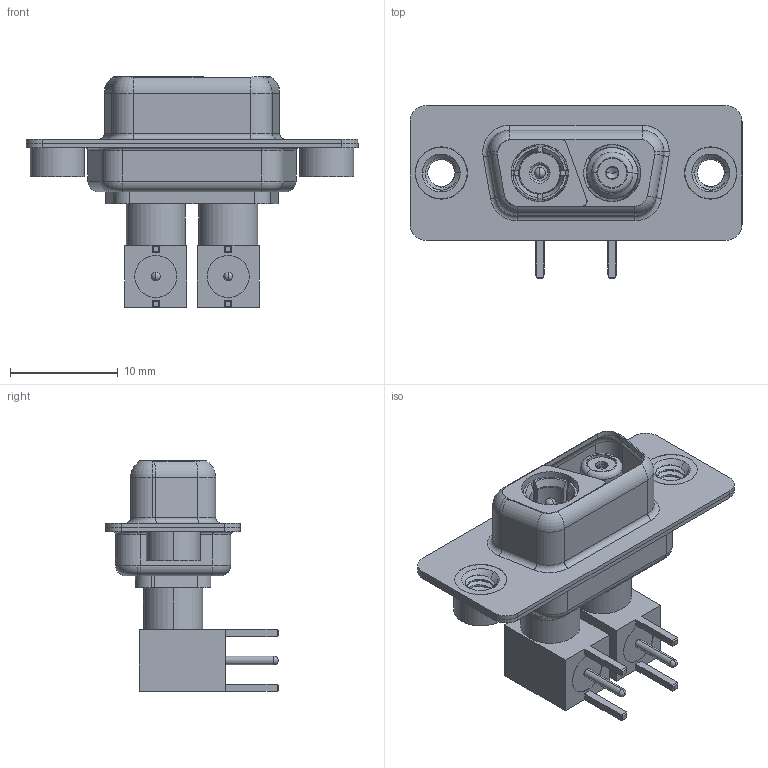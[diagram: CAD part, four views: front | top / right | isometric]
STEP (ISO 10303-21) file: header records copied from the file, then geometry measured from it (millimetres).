
FILE_DESCRIPTION (( 'STEP AP203' ), '1' );
FILE_NAME ('630-2WK2240-7TA.STEP', '2022-05-26T23:52:27', ( '' ), ( '' ), 'SwSTEP 2.0', 'SolidWorks 2020', '' );
FILE_SCHEMA (( 'CONFIG_CONTROL_DESIGN' ));
Length unit declared in the file: millimetre
Products named in the file (17): Locking Collar; 630Combo Shell Front_09 Contacts; 630Combo Housing_2WK2; Co-Ax Jack Assy_RA; Co-Ax Plug Assy_RA; Co-Ax Jack_RA PC Tail; Insulator Socket; RA Back Shell; Co-Ax Plug_RA PC Tail; Pin_RA; Insulator Pin_Straight PC Tail; Insulator Socket 2; Insulator RA Pin; 630Combo Threaded Rivet_A; 630-2WK2240-7TA; Socket_RA; 630Combo Shell Rear_09 Contacts
Assembly tree (20 placements, depth 3):
  630-2WK2240-7TA
    630Combo Housing_2WK2
    630Combo Shell Front_09 Contacts
    630Combo Shell Rear_09 Contacts
    630Combo Threaded Rivet_A  x2
    Co-Ax Plug Assy_RA
      Co-Ax Plug_RA PC Tail
      Insulator Pin_Straight PC Tail
      Pin_RA
      Locking Collar
      RA Back Shell
      Insulator RA Pin
    Co-Ax Jack Assy_RA
      Co-Ax Jack_RA PC Tail
      Insulator Socket
      Insulator Socket 2
      Locking Collar
      Socket_RA
      RA Back Shell
      Insulator RA Pin
Bounding box: 30.8 x 16 x 21.41 mm (x, y, z)
Volume: 2004.9 mm3; surface area: 5571.2 mm2
Topology: 18 solids, 18 shells, 594 faces, 1420 edges, 885 vertices
Faces by surface type: cylinder 268, plane 191, torus 69, cone 52, bspline 8, sphere 6
Entity records: 18344 total; most frequent: CARTESIAN_POINT 4417, DIRECTION 2720, ORIENTED_EDGE 2386, EDGE_CURVE 1193, AXIS2_PLACEMENT_3D 1108, VERTEX_POINT 752, CIRCLE 580, EDGE_LOOP 577
